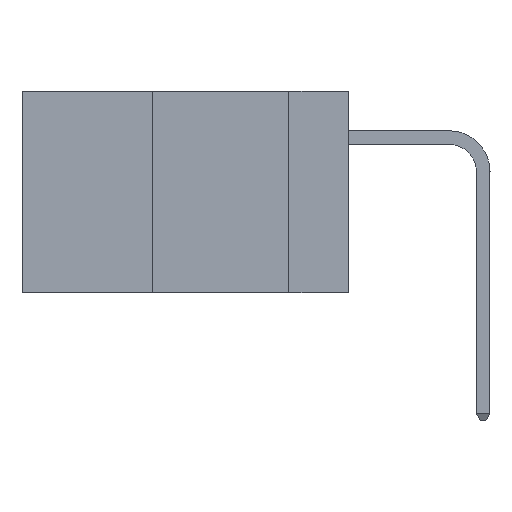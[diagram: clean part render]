
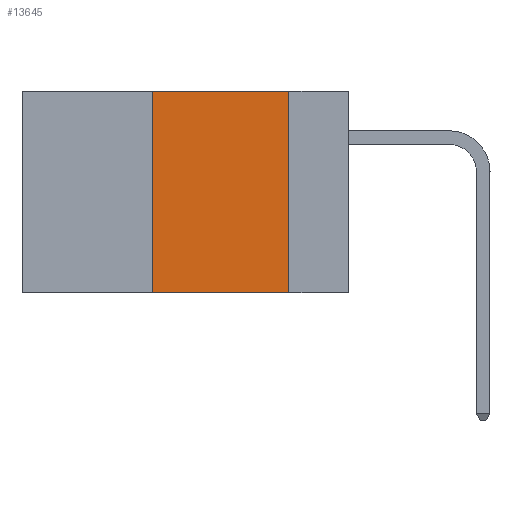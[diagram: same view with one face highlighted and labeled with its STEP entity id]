
A CAD part, left-side view. The second image highlights one B-rep face of the part: STEP entity #13645.
In plain terms, the highlighted planar face has unit normal (-1, 0, 0).
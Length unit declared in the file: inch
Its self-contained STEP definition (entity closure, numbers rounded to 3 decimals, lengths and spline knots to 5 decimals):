
#311 = PLANE ( 'NONE',  #7924 ) ;
#1320 = CARTESIAN_POINT ( 'NONE',  ( 0., 0.36, 0. ) ) ;
#1980 = EDGE_LOOP ( 'NONE', ( #16568, #9559, #10463, #7039 ) ) ;
#2159 = VECTOR ( 'NONE', #2960, 39.37008 ) ;
#2830 = LINE ( 'NONE', #15371, #18245 ) ;
#2850 = FACE_OUTER_BOUND ( 'NONE', #1980, .T. ) ;
#2960 = DIRECTION ( 'NONE',  ( 0., 0., -1. ) ) ;
#3446 = DIRECTION ( 'NONE',  ( 1., 0., 0. ) ) ;
#4604 = EDGE_CURVE ( 'NONE', #16961, #11027, #17027, .T. ) ;
#4646 = VECTOR ( 'NONE', #19456, 39.37008 ) ;
#5023 = LINE ( 'NONE', #6131, #8538 ) ;
#6131 = CARTESIAN_POINT ( 'NONE',  ( 0., 0.6, 0. ) ) ;
#6219 = LINE ( 'NONE', #11918, #2159 ) ;
#7039 = ORIENTED_EDGE ( 'NONE', *, *, #14970, .T. ) ;
#7401 = CARTESIAN_POINT ( 'NONE',  ( 0., 0.11, -0.37 ) ) ;
#7403 = VERTEX_POINT ( 'NONE', #12969 ) ;
#7593 = EDGE_CURVE ( 'NONE', #7403, #14118, #6219, .T. ) ;
#7605 = CARTESIAN_POINT ( 'NONE',  ( 0., 0.36, 0. ) ) ;
#7924 = AXIS2_PLACEMENT_3D ( 'NONE', #9397, #3446, #13880 ) ;
#8538 = VECTOR ( 'NONE', #15108, 39.37008 ) ;
#9397 = CARTESIAN_POINT ( 'NONE',  ( 0., 0.6, 0. ) ) ;
#9415 = DIRECTION ( 'NONE',  ( 0., -1., 0. ) ) ;
#9559 = ORIENTED_EDGE ( 'NONE', *, *, #12923, .F. ) ;
#10463 = ORIENTED_EDGE ( 'NONE', *, *, #4604, .F. ) ;
#11027 = VERTEX_POINT ( 'NONE', #1320 ) ;
#11918 = CARTESIAN_POINT ( 'NONE',  ( 0., 0.11, 0. ) ) ;
#12923 = EDGE_CURVE ( 'NONE', #11027, #7403, #5023, .T. ) ;
#12969 = CARTESIAN_POINT ( 'NONE',  ( 0., 0.11, 0. ) ) ;
#13645 = ADVANCED_FACE ( 'NONE', ( #2850 ), #311, .F. ) ;
#13880 = DIRECTION ( 'NONE',  ( 0., 0., -1. ) ) ;
#14118 = VERTEX_POINT ( 'NONE', #7401 ) ;
#14970 = EDGE_CURVE ( 'NONE', #16961, #14118, #2830, .T. ) ;
#15108 = DIRECTION ( 'NONE',  ( 0., -1., 0. ) ) ;
#15371 = CARTESIAN_POINT ( 'NONE',  ( 0., 0.6, -0.37 ) ) ;
#16325 = CARTESIAN_POINT ( 'NONE',  ( 0., 0.36, -0.37 ) ) ;
#16568 = ORIENTED_EDGE ( 'NONE', *, *, #7593, .F. ) ;
#16961 = VERTEX_POINT ( 'NONE', #16325 ) ;
#17027 = LINE ( 'NONE', #7605, #4646 ) ;
#18245 = VECTOR ( 'NONE', #9415, 39.37008 ) ;
#19456 = DIRECTION ( 'NONE',  ( 0., 0., 1. ) ) ;
